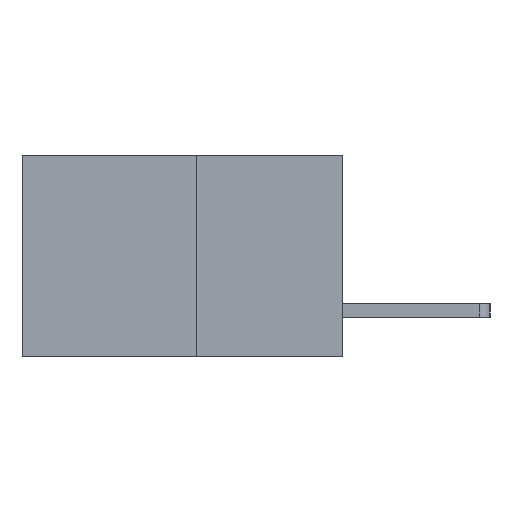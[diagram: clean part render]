
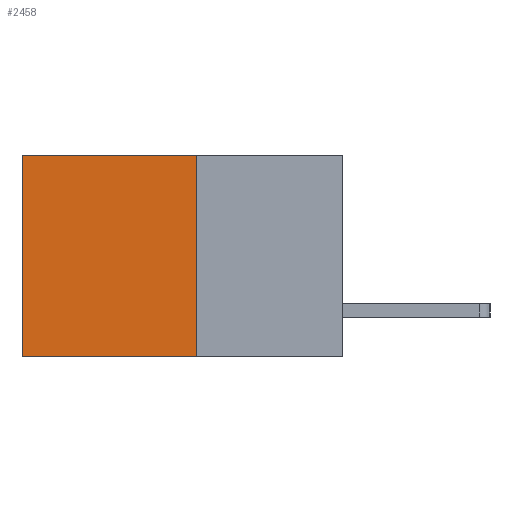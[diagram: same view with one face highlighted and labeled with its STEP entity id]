
A CAD part, left-side view. The second image highlights one B-rep face of the part: STEP entity #2458.
In plain terms, the highlighted planar face has unit normal (-1, 0, 0).
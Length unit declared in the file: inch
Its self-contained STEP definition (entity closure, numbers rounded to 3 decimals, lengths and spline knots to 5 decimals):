
#190 = DIRECTION ( 'NONE',  ( 0., 0., -1. ) ) ;
#206 = CARTESIAN_POINT ( 'NONE',  ( 0.277, 0.27, 0. ) ) ;
#233 = DIRECTION ( 'NONE',  ( 0., 1., 0. ) ) ;
#390 = LINE ( 'NONE', #206, #2402 ) ;
#684 = DIRECTION ( 'NONE',  ( 0., 0., -1. ) ) ;
#710 = ORIENTED_EDGE ( 'NONE', *, *, #5756, .T. ) ;
#747 = VECTOR ( 'NONE', #9661, 39.37008 ) ;
#1142 = ORIENTED_EDGE ( 'NONE', *, *, #6749, .F. ) ;
#1576 = CARTESIAN_POINT ( 'NONE',  ( 0.277, 0.27, -0.37 ) ) ;
#1644 = ORIENTED_EDGE ( 'NONE', *, *, #8812, .F. ) ;
#1880 = VECTOR ( 'NONE', #684, 39.37008 ) ;
#2166 = VERTEX_POINT ( 'NONE', #6405 ) ;
#2402 = VECTOR ( 'NONE', #233, 39.37008 ) ;
#2458 = ADVANCED_FACE ( 'NONE', ( #7781 ), #9470, .F. ) ;
#3013 = LINE ( 'NONE', #8300, #747 ) ;
#3149 = ORIENTED_EDGE ( 'NONE', *, *, #3529, .T. ) ;
#3329 = CARTESIAN_POINT ( 'NONE',  ( 0.277, 0.27, -0.37 ) ) ;
#3529 = EDGE_CURVE ( 'NONE', #7443, #2166, #390, .T. ) ;
#3791 = EDGE_LOOP ( 'NONE', ( #710, #1644, #1142, #3149 ) ) ;
#4363 = AXIS2_PLACEMENT_3D ( 'NONE', #1576, #8752, #10221 ) ;
#5756 = EDGE_CURVE ( 'NONE', #2166, #8251, #8030, .T. ) ;
#6238 = CARTESIAN_POINT ( 'NONE',  ( 0.277, 0.27, -0.37 ) ) ;
#6405 = CARTESIAN_POINT ( 'NONE',  ( 0.277, 0.59, 0. ) ) ;
#6749 = EDGE_CURVE ( 'NONE', #7443, #7817, #8862, .T. ) ;
#7443 = VERTEX_POINT ( 'NONE', #9638 ) ;
#7533 = VECTOR ( 'NONE', #190, 39.37008 ) ;
#7553 = CARTESIAN_POINT ( 'NONE',  ( 0.277, 0.59, -0.37 ) ) ;
#7781 = FACE_OUTER_BOUND ( 'NONE', #3791, .T. ) ;
#7817 = VERTEX_POINT ( 'NONE', #6238 ) ;
#8030 = LINE ( 'NONE', #10470, #7533 ) ;
#8251 = VERTEX_POINT ( 'NONE', #7553 ) ;
#8300 = CARTESIAN_POINT ( 'NONE',  ( 0.277, 0.27, -0.37 ) ) ;
#8752 = DIRECTION ( 'NONE',  ( 1., 0., 0. ) ) ;
#8812 = EDGE_CURVE ( 'NONE', #7817, #8251, #3013, .T. ) ;
#8862 = LINE ( 'NONE', #3329, #1880 ) ;
#9470 = PLANE ( 'NONE',  #4363 ) ;
#9638 = CARTESIAN_POINT ( 'NONE',  ( 0.277, 0.27, 0. ) ) ;
#9661 = DIRECTION ( 'NONE',  ( 0., 1., 0. ) ) ;
#10221 = DIRECTION ( 'NONE',  ( 0., 0., -1. ) ) ;
#10470 = CARTESIAN_POINT ( 'NONE',  ( 0.277, 0.59, -0.37 ) ) ;
